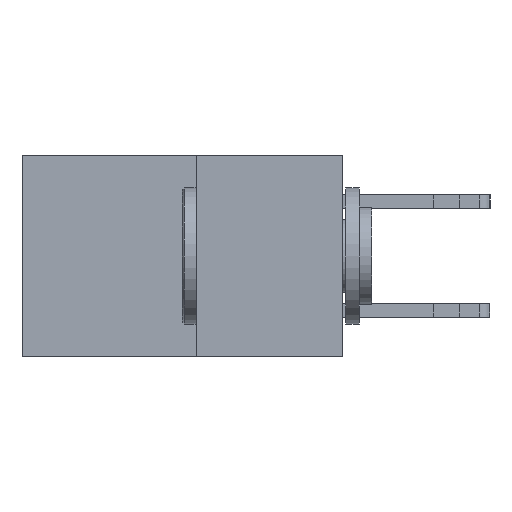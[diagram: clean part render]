
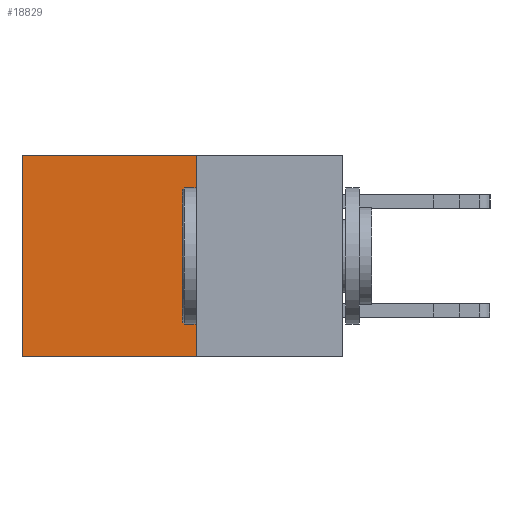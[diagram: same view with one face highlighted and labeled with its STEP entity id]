
A CAD part, left-side view. The second image highlights one B-rep face of the part: STEP entity #18829.
In plain terms, the highlighted planar face has unit normal (-1, 0, 0).
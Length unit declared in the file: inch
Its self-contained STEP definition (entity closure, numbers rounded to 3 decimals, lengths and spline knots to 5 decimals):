
#23 = CARTESIAN_POINT ( 'NONE',  ( 0.277, 0.27, -0.37 ) ) ;
#339 = FACE_OUTER_BOUND ( 'NONE', #18631, .T. ) ;
#1083 = EDGE_CURVE ( 'NONE', #12902, #13228, #20678, .T. ) ;
#2154 = CARTESIAN_POINT ( 'NONE',  ( 0.277, 0.27, 0. ) ) ;
#2380 = LINE ( 'NONE', #5187, #6914 ) ;
#3472 = EDGE_CURVE ( 'NONE', #12902, #15778, #17328, .T. ) ;
#4356 = EDGE_CURVE ( 'NONE', #15778, #22535, #21418, .T. ) ;
#5187 = CARTESIAN_POINT ( 'NONE',  ( 0.277, 0.27, -0.37 ) ) ;
#6881 = ORIENTED_EDGE ( 'NONE', *, *, #1083, .F. ) ;
#6914 = VECTOR ( 'NONE', #7154, 39.37008 ) ;
#7154 = DIRECTION ( 'NONE',  ( 0., 1., 0. ) ) ;
#7193 = DIRECTION ( 'NONE',  ( 0., 0., -1. ) ) ;
#7232 = PLANE ( 'NONE',  #15206 ) ;
#9143 = DIRECTION ( 'NONE',  ( 1., 0., 0. ) ) ;
#11827 = VECTOR ( 'NONE', #19359, 39.37008 ) ;
#12185 = CARTESIAN_POINT ( 'NONE',  ( 0.277, 0.59, 0. ) ) ;
#12902 = VERTEX_POINT ( 'NONE', #2154 ) ;
#13228 = VERTEX_POINT ( 'NONE', #18279 ) ;
#15206 = AXIS2_PLACEMENT_3D ( 'NONE', #18462, #9143, #22218 ) ;
#15684 = VECTOR ( 'NONE', #7193, 39.37008 ) ;
#15778 = VERTEX_POINT ( 'NONE', #12185 ) ;
#16021 = EDGE_CURVE ( 'NONE', #13228, #22535, #2380, .T. ) ;
#17328 = LINE ( 'NONE', #18429, #11827 ) ;
#18239 = DIRECTION ( 'NONE',  ( 0., 0., -1. ) ) ;
#18279 = CARTESIAN_POINT ( 'NONE',  ( 0.277, 0.27, -0.37 ) ) ;
#18292 = CARTESIAN_POINT ( 'NONE',  ( 0.277, 0.59, -0.37 ) ) ;
#18429 = CARTESIAN_POINT ( 'NONE',  ( 0.277, 0.27, 0. ) ) ;
#18462 = CARTESIAN_POINT ( 'NONE',  ( 0.277, 0.27, -0.37 ) ) ;
#18631 = EDGE_LOOP ( 'NONE', ( #23122, #23139, #6881, #21618 ) ) ;
#18829 = ADVANCED_FACE ( 'NONE', ( #339 ), #7232, .F. ) ;
#19359 = DIRECTION ( 'NONE',  ( 0., 1., 0. ) ) ;
#19591 = CARTESIAN_POINT ( 'NONE',  ( 0.277, 0.59, -0.37 ) ) ;
#20678 = LINE ( 'NONE', #23, #15684 ) ;
#21418 = LINE ( 'NONE', #18292, #21987 ) ;
#21618 = ORIENTED_EDGE ( 'NONE', *, *, #3472, .T. ) ;
#21987 = VECTOR ( 'NONE', #18239, 39.37008 ) ;
#22218 = DIRECTION ( 'NONE',  ( 0., 0., -1. ) ) ;
#22535 = VERTEX_POINT ( 'NONE', #19591 ) ;
#23122 = ORIENTED_EDGE ( 'NONE', *, *, #4356, .T. ) ;
#23139 = ORIENTED_EDGE ( 'NONE', *, *, #16021, .F. ) ;
